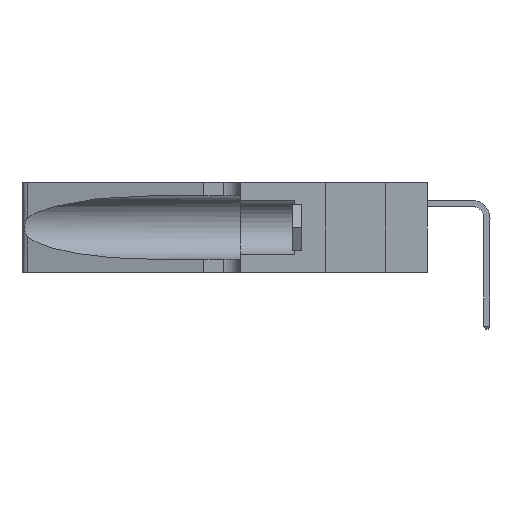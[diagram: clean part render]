
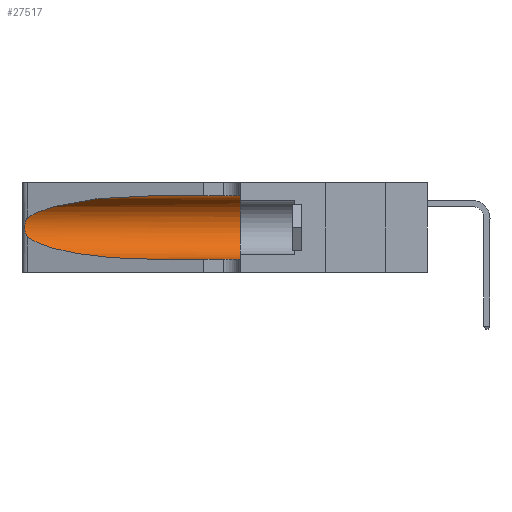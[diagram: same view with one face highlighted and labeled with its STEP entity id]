
A CAD part, left-side view. The second image highlights one B-rep face of the part: STEP entity #27517.
In plain terms, the highlighted cylindrical face has radius 3.308 mm (diameter 6.617 mm), a partial arc.
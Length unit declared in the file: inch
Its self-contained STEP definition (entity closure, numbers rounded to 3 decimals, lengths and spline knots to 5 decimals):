
#268 = ORIENTED_EDGE ( 'NONE', *, *, #15248, .T. ) ;
#1078 = DIRECTION ( 'NONE',  ( 0., 0., -1. ) ) ;
#1087 = CARTESIAN_POINT ( 'NONE',  ( 0.25639, 1.23186, 0.15144 ) ) ;
#2063 = CARTESIAN_POINT ( 'NONE',  ( 0.1305, 1.61858, 0.31525 ) ) ;
#2780 = CIRCLE ( 'NONE', #28426, 0.13025 ) ;
#3017 = CARTESIAN_POINT ( 'NONE',  ( 0.25487, 1.22718, 0.14631 ) ) ;
#3030 = ORIENTED_EDGE ( 'NONE', *, *, #16743, .F. ) ;
#3281 = CARTESIAN_POINT ( 'NONE',  ( 0.1305, 1.61858, 0.05475 ) ) ;
#3567 = CARTESIAN_POINT ( 'NONE',  ( 0.25487, 1.22718, 0.14631 ) ) ;
#3827 = CARTESIAN_POINT ( 'NONE',  ( 0.25487, 1.22718, 0.14631 ) ) ;
#4060 = ORIENTED_EDGE ( 'NONE', *, *, #18762, .T. ) ;
#5496 = VERTEX_POINT ( 'NONE', #18708 ) ;
#5965 = DIRECTION ( 'NONE',  ( 0., -1., 0. ) ) ;
#6382 = DIRECTION ( 'NONE',  ( 0., -1., 0. ) ) ;
#6399 = CARTESIAN_POINT ( 'NONE',  ( 0.25639, 1.23184, 0.21858 ) ) ;
#6740 =( BOUNDED_CURVE ( )  B_SPLINE_CURVE ( 3, ( #7021, #20398, #23101, #25764 ),
 .UNSPECIFIED., .F., .F. ) 
 B_SPLINE_CURVE_WITH_KNOTS ( ( 4, 4 ),
 ( 1.5708, 2.84003 ),
 .UNSPECIFIED. ) 
 CURVE ( )  GEOMETRIC_REPRESENTATION_ITEM ( )  RATIONAL_B_SPLINE_CURVE ( ( 1., 0.87, 0.87, 1. ) ) 
 REPRESENTATION_ITEM ( '' )  );
#7021 = CARTESIAN_POINT ( 'NONE',  ( 0.1305, 0.72297, 0.31525 ) ) ;
#9070 = CARTESIAN_POINT ( 'NONE',  ( 0.25854, 1.2359, 0.20912 ) ) ;
#9251 = VERTEX_POINT ( 'NONE', #3017 ) ;
#9971 = AXIS2_PLACEMENT_3D ( 'NONE', #17196, #6382, #1078 ) ;
#10574 = LINE ( 'NONE', #2063, #31030 ) ;
#11654 = CARTESIAN_POINT ( 'NONE',  ( 0.1305, 0.72297, 0.05475 ) ) ;
#11795 = CARTESIAN_POINT ( 'NONE',  ( 0.26075, 1.23896, 0.19203 ) ) ;
#12831 = ORIENTED_EDGE ( 'NONE', *, *, #14412, .T. ) ;
#14412 = EDGE_CURVE ( 'NONE', #29131, #26895, #6740, .T. ) ;
#14504 = CARTESIAN_POINT ( 'NONE',  ( 0.26017, 1.23833, 0.17102 ) ) ;
#14879 = ORIENTED_EDGE ( 'NONE', *, *, #18393, .F. ) ;
#15242 = FACE_OUTER_BOUND ( 'NONE', #28789, .T. ) ;
#15248 = EDGE_CURVE ( 'NONE', #9251, #5496, #16979, .T. ) ;
#15394 = CARTESIAN_POINT ( 'NONE',  ( 0.1305, 0.35, 0.185 ) ) ;
#16743 = EDGE_CURVE ( 'NONE', #29131, #18568, #10574, .T. ) ;
#16979 =( BOUNDED_CURVE ( )  B_SPLINE_CURVE ( 3, ( #3567, #19644, #27667, #11654 ),
 .UNSPECIFIED., .F., .F. ) 
 B_SPLINE_CURVE_WITH_KNOTS ( ( 4, 4 ),
 ( 3.44316, 4.71239 ),
 .UNSPECIFIED. ) 
 CURVE ( )  GEOMETRIC_REPRESENTATION_ITEM ( )  RATIONAL_B_SPLINE_CURVE ( ( 1., 0.87, 0.87, 1. ) ) 
 REPRESENTATION_ITEM ( '' )  );
#17196 = CARTESIAN_POINT ( 'NONE',  ( 0.1305, 1.61858, 0.185 ) ) ;
#17214 = CARTESIAN_POINT ( 'NONE',  ( 0.25789, 1.23486, 0.15765 ) ) ;
#18096 = DIRECTION ( 'NONE',  ( 0., 0., 1. ) ) ;
#18393 = EDGE_CURVE ( 'NONE', #18568, #24509, #2780, .T. ) ;
#18511 = CARTESIAN_POINT ( 'NONE',  ( 0.1305, 0.72297, 0.31525 ) ) ;
#18568 = VERTEX_POINT ( 'NONE', #21362 ) ;
#18708 = CARTESIAN_POINT ( 'NONE',  ( 0.1305, 0.72297, 0.05475 ) ) ;
#18762 = EDGE_CURVE ( 'NONE', #5496, #24509, #33656, .T. ) ;
#19420 = EDGE_CURVE ( 'NONE', #26895, #9251, #29621, .T. ) ;
#19644 = CARTESIAN_POINT ( 'NONE',  ( 0.2373, 1.15595, 0.08982 ) ) ;
#19786 = CARTESIAN_POINT ( 'NONE',  ( 0.25487, 1.22718, 0.22369 ) ) ;
#19902 = CARTESIAN_POINT ( 'NONE',  ( 0.25555, 1.22993, 0.14849 ) ) ;
#20398 = CARTESIAN_POINT ( 'NONE',  ( 0.18966, 0.96281, 0.31525 ) ) ;
#21362 = CARTESIAN_POINT ( 'NONE',  ( 0.1305, 0.35, 0.31525 ) ) ;
#22050 = VECTOR ( 'NONE', #5965, 39.37008 ) ;
#22991 = ORIENTED_EDGE ( 'NONE', *, *, #19420, .T. ) ;
#23101 = CARTESIAN_POINT ( 'NONE',  ( 0.2373, 1.15595, 0.28018 ) ) ;
#24509 = VERTEX_POINT ( 'NONE', #26198 ) ;
#25162 = CARTESIAN_POINT ( 'NONE',  ( 0.25787, 1.23484, 0.2124 ) ) ;
#25764 = CARTESIAN_POINT ( 'NONE',  ( 0.25487, 1.22718, 0.22369 ) ) ;
#26198 = CARTESIAN_POINT ( 'NONE',  ( 0.1305, 0.35, 0.05475 ) ) ;
#26895 = VERTEX_POINT ( 'NONE', #27493 ) ;
#27493 = CARTESIAN_POINT ( 'NONE',  ( 0.25487, 1.22718, 0.22369 ) ) ;
#27517 = ADVANCED_FACE ( 'NONE', ( #15242 ), #28605, .F. ) ;
#27667 = CARTESIAN_POINT ( 'NONE',  ( 0.18966, 0.96281, 0.05475 ) ) ;
#27698 = CARTESIAN_POINT ( 'NONE',  ( 0.25555, 1.22994, 0.2215 ) ) ;
#27815 = CARTESIAN_POINT ( 'NONE',  ( 0.26018, 1.23835, 0.19895 ) ) ;
#28426 = AXIS2_PLACEMENT_3D ( 'NONE', #15394, #33979, #18096 ) ;
#28605 = CYLINDRICAL_SURFACE ( 'NONE', #9971, 0.13025 ) ;
#28789 = EDGE_LOOP ( 'NONE', ( #12831, #22991, #268, #4060, #14879, #3030 ) ) ;
#29131 = VERTEX_POINT ( 'NONE', #18511 ) ;
#29621 = B_SPLINE_CURVE_WITH_KNOTS ( 'NONE', 3,
 ( #19786, #27698, #6399, #25162, #9070, #27815, #11795, #30477, #14504, #33120, #17214, #1087, #19902, #3827 ),
 .UNSPECIFIED., .F., .F.,
 ( 4, 2, 2, 2, 2, 2, 4 ),
 ( 0., 0.00027, 0.00053, 0.00107, 0.0016, 0.00187, 0.00214 ),
 .UNSPECIFIED. ) ;
#30477 = CARTESIAN_POINT ( 'NONE',  ( 0.26075, 1.23896, 0.178 ) ) ;
#31030 = VECTOR ( 'NONE', #34039, 39.37008 ) ;
#33120 = CARTESIAN_POINT ( 'NONE',  ( 0.25856, 1.23593, 0.16098 ) ) ;
#33656 = LINE ( 'NONE', #3281, #22050 ) ;
#33979 = DIRECTION ( 'NONE',  ( 0., 1., 0. ) ) ;
#34039 = DIRECTION ( 'NONE',  ( 0., -1., 0. ) ) ;
